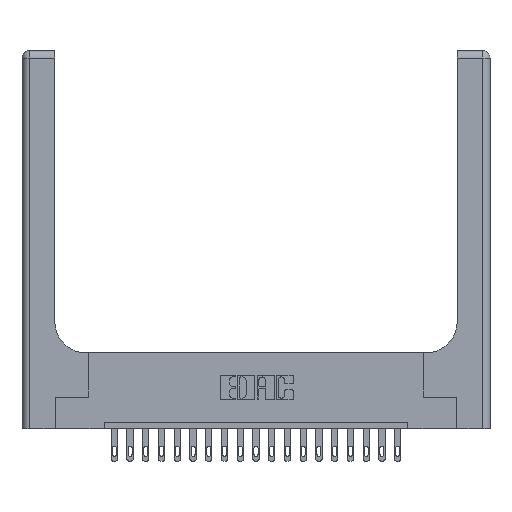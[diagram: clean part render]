
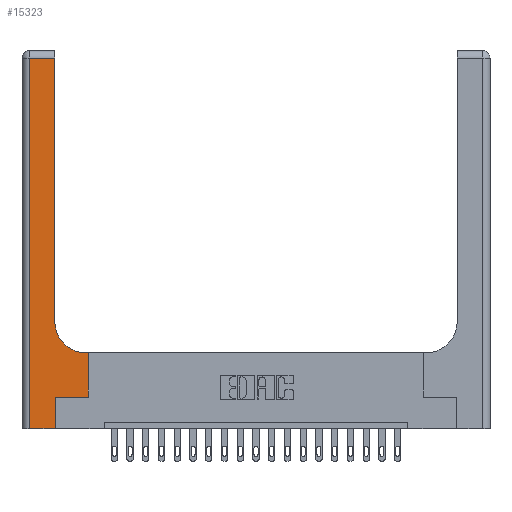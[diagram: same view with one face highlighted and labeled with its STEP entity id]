
A CAD part, top view. The second image highlights one B-rep face of the part: STEP entity #15323.
In plain terms, the highlighted planar face has unit normal (0, 0, 1).
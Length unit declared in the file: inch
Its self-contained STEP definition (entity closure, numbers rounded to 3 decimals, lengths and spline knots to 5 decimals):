
#307 = LINE ( 'NONE', #6613, #5209 ) ;
#613 = ORIENTED_EDGE ( 'NONE', *, *, #9278, .T. ) ;
#797 = VECTOR ( 'NONE', #15019, 39.37008 ) ;
#879 = CARTESIAN_POINT ( 'NONE',  ( 0., 0., 0.37 ) ) ;
#1054 = DIRECTION ( 'NONE',  ( 0., 1., 0. ) ) ;
#1075 = EDGE_CURVE ( 'NONE', #19295, #19456, #19380, .T. ) ;
#1203 = VERTEX_POINT ( 'NONE', #18238 ) ;
#1255 = CARTESIAN_POINT ( 'NONE',  ( 0.265, 0., 0.37 ) ) ;
#2013 = PLANE ( 'NONE',  #10187 ) ;
#2236 = VECTOR ( 'NONE', #5239, 39.37008 ) ;
#3021 = ORIENTED_EDGE ( 'NONE', *, *, #18052, .T. ) ;
#3301 = EDGE_CURVE ( 'NONE', #19456, #12234, #12008, .T. ) ;
#3839 = VECTOR ( 'NONE', #4154, 39.37008 ) ;
#3859 = LINE ( 'NONE', #17791, #797 ) ;
#4154 = DIRECTION ( 'NONE',  ( 0., -1., 0. ) ) ;
#4162 = LINE ( 'NONE', #15226, #18141 ) ;
#4696 = CARTESIAN_POINT ( 'NONE',  ( 0.51, 0.6, 0.37 ) ) ;
#5027 = DIRECTION ( 'NONE',  ( 0., 1., 0. ) ) ;
#5209 = VECTOR ( 'NONE', #11366, 39.37008 ) ;
#5239 = DIRECTION ( 'NONE',  ( -1., 0., 0. ) ) ;
#5473 = CIRCLE ( 'NONE', #12407, 0.25 ) ;
#5509 = CARTESIAN_POINT ( 'NONE',  ( 0.06, 2.94, 0.37 ) ) ;
#5740 = LINE ( 'NONE', #879, #16740 ) ;
#5835 = VERTEX_POINT ( 'NONE', #9510 ) ;
#6094 = CARTESIAN_POINT ( 'NONE',  ( 0.06, 0., 0.37 ) ) ;
#6613 = CARTESIAN_POINT ( 'NONE',  ( 0.265, 0.25, 0.37 ) ) ;
#6677 = CARTESIAN_POINT ( 'NONE',  ( 0., 2.94, 0.37 ) ) ;
#7201 = VERTEX_POINT ( 'NONE', #4696 ) ;
#7443 = VERTEX_POINT ( 'NONE', #1255 ) ;
#7696 = DIRECTION ( 'NONE',  ( 1., 0., 0. ) ) ;
#7981 = CARTESIAN_POINT ( 'NONE',  ( 0.26, 2.94, 0.37 ) ) ;
#9278 = EDGE_CURVE ( 'NONE', #7201, #1203, #5473, .T. ) ;
#9510 = CARTESIAN_POINT ( 'NONE',  ( 0.528, 0.25, 0.37 ) ) ;
#9775 = CARTESIAN_POINT ( 'NONE',  ( 0., 3., 0.37 ) ) ;
#9873 = VECTOR ( 'NONE', #5027, 39.37008 ) ;
#10176 = DIRECTION ( 'NONE',  ( 1., 0., 0. ) ) ;
#10187 = AXIS2_PLACEMENT_3D ( 'NONE', #9775, #17921, #14735 ) ;
#10598 = DIRECTION ( 'NONE',  ( 0., 0., -1. ) ) ;
#10615 = ORIENTED_EDGE ( 'NONE', *, *, #12852, .T. ) ;
#11366 = DIRECTION ( 'NONE',  ( 1., 0., 0. ) ) ;
#11734 = FACE_OUTER_BOUND ( 'NONE', #20143, .T. ) ;
#12008 = LINE ( 'NONE', #18297, #3839 ) ;
#12234 = VERTEX_POINT ( 'NONE', #6094 ) ;
#12293 = CARTESIAN_POINT ( 'NONE',  ( 0.265, 0.25, 0.37 ) ) ;
#12407 = AXIS2_PLACEMENT_3D ( 'NONE', #20011, #10598, #7696 ) ;
#12852 = EDGE_CURVE ( 'NONE', #14331, #7201, #3859, .T. ) ;
#13719 = LINE ( 'NONE', #20021, #15485 ) ;
#13855 = ORIENTED_EDGE ( 'NONE', *, *, #1075, .T. ) ;
#13867 = ORIENTED_EDGE ( 'NONE', *, *, #3301, .T. ) ;
#14252 = EDGE_CURVE ( 'NONE', #12234, #7443, #5740, .T. ) ;
#14331 = VERTEX_POINT ( 'NONE', #16879 ) ;
#14432 = LINE ( 'NONE', #19170, #9873 ) ;
#14735 = DIRECTION ( 'NONE',  ( -1., 0., 0. ) ) ;
#15019 = DIRECTION ( 'NONE',  ( -1., 0., 0. ) ) ;
#15226 = CARTESIAN_POINT ( 'NONE',  ( 0.265, 0., 0.37 ) ) ;
#15323 = ADVANCED_FACE ( 'NONE', ( #11734 ), #2013, .F. ) ;
#15485 = VECTOR ( 'NONE', #16897, 39.37008 ) ;
#15988 = EDGE_CURVE ( 'NONE', #16158, #5835, #307, .T. ) ;
#16158 = VERTEX_POINT ( 'NONE', #12293 ) ;
#16575 = ORIENTED_EDGE ( 'NONE', *, *, #14252, .T. ) ;
#16713 = EDGE_CURVE ( 'NONE', #5835, #14331, #13719, .T. ) ;
#16740 = VECTOR ( 'NONE', #10176, 39.37008 ) ;
#16879 = CARTESIAN_POINT ( 'NONE',  ( 0.528, 0.6, 0.37 ) ) ;
#16897 = DIRECTION ( 'NONE',  ( 0., 1., 0. ) ) ;
#17312 = ORIENTED_EDGE ( 'NONE', *, *, #18677, .T. ) ;
#17791 = CARTESIAN_POINT ( 'NONE',  ( 0.26, 0.6, 0.37 ) ) ;
#17921 = DIRECTION ( 'NONE',  ( 0., 0., -1. ) ) ;
#18052 = EDGE_CURVE ( 'NONE', #1203, #19295, #14432, .T. ) ;
#18141 = VECTOR ( 'NONE', #1054, 39.37008 ) ;
#18238 = CARTESIAN_POINT ( 'NONE',  ( 0.26, 0.85, 0.37 ) ) ;
#18297 = CARTESIAN_POINT ( 'NONE',  ( 0.06, 3., 0.37 ) ) ;
#18677 = EDGE_CURVE ( 'NONE', #7443, #16158, #4162, .T. ) ;
#19170 = CARTESIAN_POINT ( 'NONE',  ( 0.26, 3., 0.37 ) ) ;
#19295 = VERTEX_POINT ( 'NONE', #7981 ) ;
#19380 = LINE ( 'NONE', #6677, #2236 ) ;
#19427 = ORIENTED_EDGE ( 'NONE', *, *, #15988, .T. ) ;
#19456 = VERTEX_POINT ( 'NONE', #5509 ) ;
#19765 = ORIENTED_EDGE ( 'NONE', *, *, #16713, .T. ) ;
#20011 = CARTESIAN_POINT ( 'NONE',  ( 0.51, 0.85, 0.37 ) ) ;
#20021 = CARTESIAN_POINT ( 'NONE',  ( 0.528, 0.25, 0.37 ) ) ;
#20143 = EDGE_LOOP ( 'NONE', ( #3021, #13855, #13867, #16575, #17312, #19427, #19765, #10615, #613 ) ) ;
